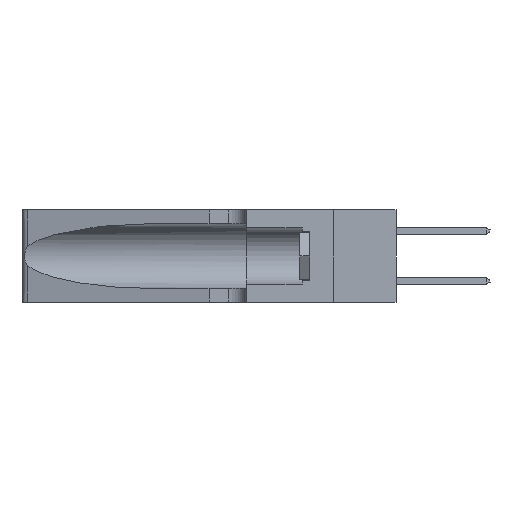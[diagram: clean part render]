
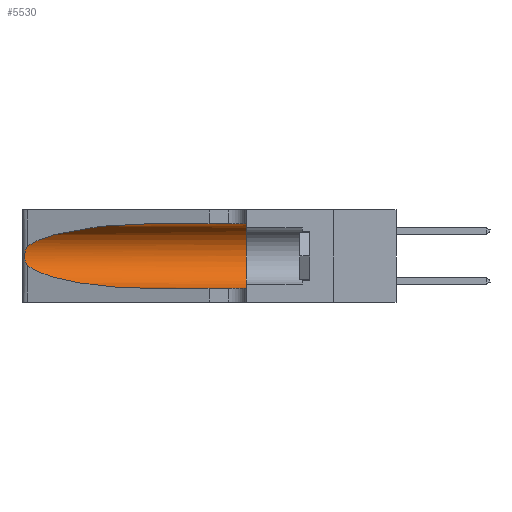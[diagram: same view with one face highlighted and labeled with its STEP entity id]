
A CAD part, left-side view. The second image highlights one B-rep face of the part: STEP entity #5530.
In plain terms, the highlighted cylindrical face has radius 3.308 mm (diameter 6.617 mm), a partial arc.
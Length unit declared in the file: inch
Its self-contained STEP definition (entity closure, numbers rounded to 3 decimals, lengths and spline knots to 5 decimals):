
#1406 = VECTOR ( 'NONE', #22435, 39.37008 ) ;
#1719 = CARTESIAN_POINT ( 'NONE',  ( 0.25639, 1.23186, 0.15144 ) ) ;
#1744 = CARTESIAN_POINT ( 'NONE',  ( 0.25487, 1.22718, 0.22369 ) ) ;
#3055 = CARTESIAN_POINT ( 'NONE',  ( 0.1305, 0.35, 0.31525 ) ) ;
#3427 = AXIS2_PLACEMENT_3D ( 'NONE', #14515, #17983, #22345 ) ;
#3775 = ORIENTED_EDGE ( 'NONE', *, *, #9131, .F. ) ;
#4467 = VERTEX_POINT ( 'NONE', #3055 ) ;
#4766 = ORIENTED_EDGE ( 'NONE', *, *, #17624, .F. ) ;
#5067 = CARTESIAN_POINT ( 'NONE',  ( 0.25854, 1.2359, 0.20912 ) ) ;
#5073 = ORIENTED_EDGE ( 'NONE', *, *, #24015, .T. ) ;
#5242 = CARTESIAN_POINT ( 'NONE',  ( 0.25487, 1.22718, 0.14631 ) ) ;
#5517 = CARTESIAN_POINT ( 'NONE',  ( 0.25555, 1.22993, 0.14849 ) ) ;
#5530 = ADVANCED_FACE ( 'NONE', ( #38193 ), #40404, .F. ) ;
#6804 =( BOUNDED_CURVE ( )  B_SPLINE_CURVE ( 3, ( #15248, #28168, #28469, #1744 ),
 .UNSPECIFIED., .F., .F. ) 
 B_SPLINE_CURVE_WITH_KNOTS ( ( 4, 4 ),
 ( 1.5708, 2.84003 ),
 .UNSPECIFIED. ) 
 CURVE ( )  GEOMETRIC_REPRESENTATION_ITEM ( )  RATIONAL_B_SPLINE_CURVE ( ( 1., 0.87, 0.87, 1. ) ) 
 REPRESENTATION_ITEM ( '' )  );
#7327 = LINE ( 'NONE', #22285, #1406 ) ;
#8844 = ORIENTED_EDGE ( 'NONE', *, *, #14393, .T. ) ;
#9131 = EDGE_CURVE ( 'NONE', #4467, #18191, #17473, .T. ) ;
#9166 = ORIENTED_EDGE ( 'NONE', *, *, #10626, .T. ) ;
#9596 = CARTESIAN_POINT ( 'NONE',  ( 0.25487, 1.22718, 0.14631 ) ) ;
#10502 = VERTEX_POINT ( 'NONE', #37814 ) ;
#10626 = EDGE_CURVE ( 'NONE', #18614, #20120, #6804, .T. ) ;
#13608 = VERTEX_POINT ( 'NONE', #20976 ) ;
#14393 = EDGE_CURVE ( 'NONE', #20120, #13608, #20792, .T. ) ;
#14515 = CARTESIAN_POINT ( 'NONE',  ( 0.1305, 0.35, 0.185 ) ) ;
#15248 = CARTESIAN_POINT ( 'NONE',  ( 0.1305, 0.72297, 0.31525 ) ) ;
#16177 = CARTESIAN_POINT ( 'NONE',  ( 0.1305, 0.72297, 0.05475 ) ) ;
#17473 = CIRCLE ( 'NONE', #3427, 0.13025 ) ;
#17624 = EDGE_CURVE ( 'NONE', #18614, #4467, #7327, .T. ) ;
#17983 = DIRECTION ( 'NONE',  ( 0., 1., 0. ) ) ;
#18191 = VERTEX_POINT ( 'NONE', #25265 ) ;
#18490 = LINE ( 'NONE', #40317, #35525 ) ;
#18614 = VERTEX_POINT ( 'NONE', #24806 ) ;
#20120 = VERTEX_POINT ( 'NONE', #42767 ) ;
#20792 = B_SPLINE_CURVE_WITH_KNOTS ( 'NONE', 3,
 ( #29514, #22263, #35779, #25502, #5067, #28908, #25941, #29361, #36079, #32524, #25788, #1719, #5517, #5242 ),
 .UNSPECIFIED., .F., .F.,
 ( 4, 2, 2, 2, 2, 2, 4 ),
 ( 0., 0.00027, 0.00053, 0.00107, 0.0016, 0.00187, 0.00214 ),
 .UNSPECIFIED. ) ;
#20976 = CARTESIAN_POINT ( 'NONE',  ( 0.25487, 1.22718, 0.14631 ) ) ;
#22263 = CARTESIAN_POINT ( 'NONE',  ( 0.25555, 1.22994, 0.2215 ) ) ;
#22285 = CARTESIAN_POINT ( 'NONE',  ( 0.1305, 1.61858, 0.31525 ) ) ;
#22345 = DIRECTION ( 'NONE',  ( 0., 0., 1. ) ) ;
#22435 = DIRECTION ( 'NONE',  ( 0., -1., 0. ) ) ;
#24015 = EDGE_CURVE ( 'NONE', #13608, #10502, #39388, .T. ) ;
#24806 = CARTESIAN_POINT ( 'NONE',  ( 0.1305, 0.72297, 0.31525 ) ) ;
#25127 = ORIENTED_EDGE ( 'NONE', *, *, #36431, .T. ) ;
#25265 = CARTESIAN_POINT ( 'NONE',  ( 0.1305, 0.35, 0.05475 ) ) ;
#25502 = CARTESIAN_POINT ( 'NONE',  ( 0.25787, 1.23484, 0.2124 ) ) ;
#25788 = CARTESIAN_POINT ( 'NONE',  ( 0.25789, 1.23486, 0.15765 ) ) ;
#25941 = CARTESIAN_POINT ( 'NONE',  ( 0.26075, 1.23896, 0.19203 ) ) ;
#26393 = DIRECTION ( 'NONE',  ( 0., -1., 0. ) ) ;
#27384 = DIRECTION ( 'NONE',  ( 0., 0., -1. ) ) ;
#28168 = CARTESIAN_POINT ( 'NONE',  ( 0.18966, 0.96281, 0.31525 ) ) ;
#28469 = CARTESIAN_POINT ( 'NONE',  ( 0.2373, 1.15595, 0.28018 ) ) ;
#28908 = CARTESIAN_POINT ( 'NONE',  ( 0.26018, 1.23835, 0.19895 ) ) ;
#29361 = CARTESIAN_POINT ( 'NONE',  ( 0.26075, 1.23896, 0.178 ) ) ;
#29514 = CARTESIAN_POINT ( 'NONE',  ( 0.25487, 1.22718, 0.22369 ) ) ;
#30417 = DIRECTION ( 'NONE',  ( 0., -1., 0. ) ) ;
#32524 = CARTESIAN_POINT ( 'NONE',  ( 0.25856, 1.23593, 0.16098 ) ) ;
#33471 = CARTESIAN_POINT ( 'NONE',  ( 0.18966, 0.96281, 0.05475 ) ) ;
#35525 = VECTOR ( 'NONE', #26393, 39.37008 ) ;
#35582 = EDGE_LOOP ( 'NONE', ( #9166, #8844, #5073, #25127, #3775, #4766 ) ) ;
#35779 = CARTESIAN_POINT ( 'NONE',  ( 0.25639, 1.23184, 0.21858 ) ) ;
#36079 = CARTESIAN_POINT ( 'NONE',  ( 0.26017, 1.23833, 0.17102 ) ) ;
#36404 = CARTESIAN_POINT ( 'NONE',  ( 0.1305, 1.61858, 0.185 ) ) ;
#36431 = EDGE_CURVE ( 'NONE', #10502, #18191, #18490, .T. ) ;
#37814 = CARTESIAN_POINT ( 'NONE',  ( 0.1305, 0.72297, 0.05475 ) ) ;
#38193 = FACE_OUTER_BOUND ( 'NONE', #35582, .T. ) ;
#38382 = AXIS2_PLACEMENT_3D ( 'NONE', #36404, #30417, #27384 ) ;
#39388 =( BOUNDED_CURVE ( )  B_SPLINE_CURVE ( 3, ( #9596, #40210, #33471, #16177 ),
 .UNSPECIFIED., .F., .F. ) 
 B_SPLINE_CURVE_WITH_KNOTS ( ( 4, 4 ),
 ( 3.44316, 4.71239 ),
 .UNSPECIFIED. ) 
 CURVE ( )  GEOMETRIC_REPRESENTATION_ITEM ( )  RATIONAL_B_SPLINE_CURVE ( ( 1., 0.87, 0.87, 1. ) ) 
 REPRESENTATION_ITEM ( '' )  );
#40210 = CARTESIAN_POINT ( 'NONE',  ( 0.2373, 1.15595, 0.08982 ) ) ;
#40317 = CARTESIAN_POINT ( 'NONE',  ( 0.1305, 1.61858, 0.05475 ) ) ;
#40404 = CYLINDRICAL_SURFACE ( 'NONE', #38382, 0.13025 ) ;
#42767 = CARTESIAN_POINT ( 'NONE',  ( 0.25487, 1.22718, 0.22369 ) ) ;
